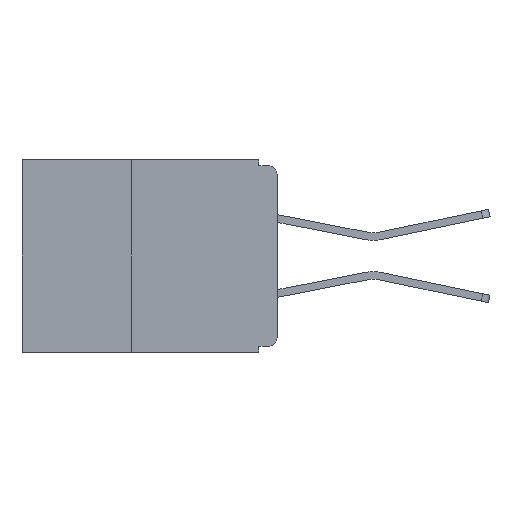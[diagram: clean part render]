
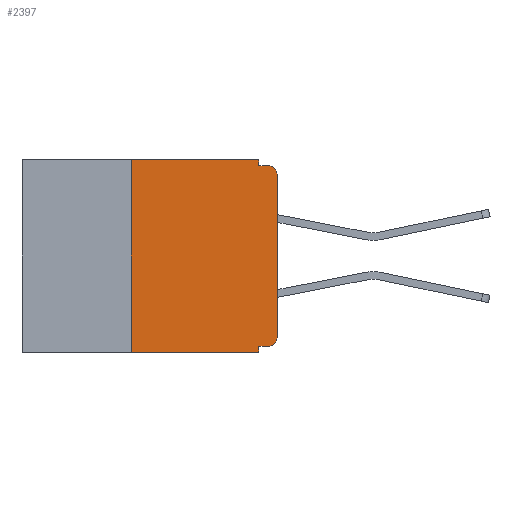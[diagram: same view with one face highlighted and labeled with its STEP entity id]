
A CAD part, left-side view. The second image highlights one B-rep face of the part: STEP entity #2397.
In plain terms, the highlighted planar face has unit normal (-1, 0, 0).
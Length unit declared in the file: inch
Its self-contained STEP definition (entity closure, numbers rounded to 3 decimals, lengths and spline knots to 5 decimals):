
#130 = VERTEX_POINT ( 'NONE', #9236 ) ;
#226 = CARTESIAN_POINT ( 'NONE',  ( 0., 0.031, -0.32 ) ) ;
#652 = EDGE_LOOP ( 'NONE', ( #1715, #4496, #15395, #12072, #7033, #8301, #9974, #15244, #3647, #6805 ) ) ;
#785 = LINE ( 'NONE', #13128, #4034 ) ;
#1080 = DIRECTION ( 'NONE',  ( 0., 0., -1. ) ) ;
#1181 = VERTEX_POINT ( 'NONE', #7535 ) ;
#1207 = LINE ( 'NONE', #7758, #7220 ) ;
#1547 = LINE ( 'NONE', #9650, #10556 ) ;
#1715 = ORIENTED_EDGE ( 'NONE', *, *, #8764, .T. ) ;
#1827 = CARTESIAN_POINT ( 'NONE',  ( 0., 0.25, 0. ) ) ;
#1903 = EDGE_CURVE ( 'NONE', #8548, #1181, #4056, .T. ) ;
#2397 = ADVANCED_FACE ( 'NONE', ( #12766 ), #10841, .F. ) ;
#3008 = DIRECTION ( 'NONE',  ( -1., 0., 0. ) ) ;
#3220 = VERTEX_POINT ( 'NONE', #9824 ) ;
#3463 = LINE ( 'NONE', #8018, #9416 ) ;
#3647 = ORIENTED_EDGE ( 'NONE', *, *, #13875, .F. ) ;
#4034 = VECTOR ( 'NONE', #11919, 39.37008 ) ;
#4056 = CIRCLE ( 'NONE', #10713, 0.015 ) ;
#4493 = DIRECTION ( 'NONE',  ( 0., -1., 0. ) ) ;
#4496 = ORIENTED_EDGE ( 'NONE', *, *, #1903, .T. ) ;
#4923 = DIRECTION ( 'NONE',  ( 0., 1., 0. ) ) ;
#5971 = CARTESIAN_POINT ( 'NONE',  ( 0., 0.25, -0.33 ) ) ;
#6262 = DIRECTION ( 'NONE',  ( 0., -1., 0. ) ) ;
#6475 = CARTESIAN_POINT ( 'NONE',  ( 0., 0.437, 0. ) ) ;
#6805 = ORIENTED_EDGE ( 'NONE', *, *, #13132, .T. ) ;
#6872 = VECTOR ( 'NONE', #4493, 39.37008 ) ;
#7033 = ORIENTED_EDGE ( 'NONE', *, *, #9371, .F. ) ;
#7164 = DIRECTION ( 'NONE',  ( 0., 0., 1. ) ) ;
#7220 = VECTOR ( 'NONE', #7387, 39.37008 ) ;
#7387 = DIRECTION ( 'NONE',  ( 0., 0., 1. ) ) ;
#7422 = VERTEX_POINT ( 'NONE', #12065 ) ;
#7535 = CARTESIAN_POINT ( 'NONE',  ( 0., 0.015, -0.01 ) ) ;
#7758 = CARTESIAN_POINT ( 'NONE',  ( 0., 0., 0. ) ) ;
#7899 = CARTESIAN_POINT ( 'NONE',  ( 0., 0.031, -0.33 ) ) ;
#7914 = LINE ( 'NONE', #8439, #13851 ) ;
#8018 = CARTESIAN_POINT ( 'NONE',  ( 0., 0.437, 0. ) ) ;
#8141 = LINE ( 'NONE', #12176, #10944 ) ;
#8180 = DIRECTION ( 'NONE',  ( 0., 0., -1. ) ) ;
#8251 = DIRECTION ( 'NONE',  ( -1., 0., 0. ) ) ;
#8301 = ORIENTED_EDGE ( 'NONE', *, *, #12025, .F. ) ;
#8344 = LINE ( 'NONE', #5971, #14274 ) ;
#8439 = CARTESIAN_POINT ( 'NONE',  ( 0., 0.031, -0.33 ) ) ;
#8548 = VERTEX_POINT ( 'NONE', #12928 ) ;
#8764 = EDGE_CURVE ( 'NONE', #3220, #8548, #1207, .T. ) ;
#9236 = CARTESIAN_POINT ( 'NONE',  ( 0., 0.25, -0.33 ) ) ;
#9352 = CARTESIAN_POINT ( 'NONE',  ( 0., 0.015, -0.32 ) ) ;
#9371 = EDGE_CURVE ( 'NONE', #9870, #7422, #3463, .T. ) ;
#9416 = VECTOR ( 'NONE', #13934, 39.37008 ) ;
#9527 = AXIS2_PLACEMENT_3D ( 'NONE', #15264, #8251, #1080 ) ;
#9545 = EDGE_CURVE ( 'NONE', #7422, #14293, #785, .T. ) ;
#9650 = CARTESIAN_POINT ( 'NONE',  ( 0., 0., -0.32 ) ) ;
#9824 = CARTESIAN_POINT ( 'NONE',  ( 0., 0., -0.305 ) ) ;
#9870 = VERTEX_POINT ( 'NONE', #1827 ) ;
#9974 = ORIENTED_EDGE ( 'NONE', *, *, #12735, .T. ) ;
#10348 = VERTEX_POINT ( 'NONE', #226 ) ;
#10394 = CARTESIAN_POINT ( 'NONE',  ( 0., 0., -0.01 ) ) ;
#10556 = VECTOR ( 'NONE', #4923, 39.37008 ) ;
#10713 = AXIS2_PLACEMENT_3D ( 'NONE', #13284, #3008, #8180 ) ;
#10841 = PLANE ( 'NONE',  #11127 ) ;
#10944 = VECTOR ( 'NONE', #6262, 39.37008 ) ;
#11127 = AXIS2_PLACEMENT_3D ( 'NONE', #6475, #12565, #12724 ) ;
#11919 = DIRECTION ( 'NONE',  ( 0., 0., -1. ) ) ;
#12025 = EDGE_CURVE ( 'NONE', #130, #9870, #8344, .T. ) ;
#12052 = CIRCLE ( 'NONE', #9527, 0.015 ) ;
#12065 = CARTESIAN_POINT ( 'NONE',  ( 0., 0.031, 0. ) ) ;
#12072 = ORIENTED_EDGE ( 'NONE', *, *, #9545, .F. ) ;
#12176 = CARTESIAN_POINT ( 'NONE',  ( 0., 0.437, -0.33 ) ) ;
#12565 = DIRECTION ( 'NONE',  ( 1., 0., 0. ) ) ;
#12724 = DIRECTION ( 'NONE',  ( 0., 0., -1. ) ) ;
#12735 = EDGE_CURVE ( 'NONE', #130, #12971, #8141, .T. ) ;
#12766 = FACE_OUTER_BOUND ( 'NONE', #652, .T. ) ;
#12928 = CARTESIAN_POINT ( 'NONE',  ( 0., 0., -0.025 ) ) ;
#12971 = VERTEX_POINT ( 'NONE', #7899 ) ;
#13032 = EDGE_CURVE ( 'NONE', #14293, #1181, #13171, .T. ) ;
#13083 = VERTEX_POINT ( 'NONE', #9352 ) ;
#13128 = CARTESIAN_POINT ( 'NONE',  ( 0., 0.031, 0. ) ) ;
#13132 = EDGE_CURVE ( 'NONE', #13083, #3220, #12052, .T. ) ;
#13171 = LINE ( 'NONE', #10394, #6872 ) ;
#13255 = DIRECTION ( 'NONE',  ( 0., 0., -1. ) ) ;
#13284 = CARTESIAN_POINT ( 'NONE',  ( 0., 0.015, -0.025 ) ) ;
#13851 = VECTOR ( 'NONE', #13255, 39.37008 ) ;
#13875 = EDGE_CURVE ( 'NONE', #13083, #10348, #1547, .T. ) ;
#13934 = DIRECTION ( 'NONE',  ( 0., -1., 0. ) ) ;
#14015 = CARTESIAN_POINT ( 'NONE',  ( 0., 0.031, -0.01 ) ) ;
#14274 = VECTOR ( 'NONE', #7164, 39.37008 ) ;
#14293 = VERTEX_POINT ( 'NONE', #14015 ) ;
#14939 = EDGE_CURVE ( 'NONE', #10348, #12971, #7914, .T. ) ;
#15244 = ORIENTED_EDGE ( 'NONE', *, *, #14939, .F. ) ;
#15264 = CARTESIAN_POINT ( 'NONE',  ( 0., 0.015, -0.305 ) ) ;
#15395 = ORIENTED_EDGE ( 'NONE', *, *, #13032, .F. ) ;
